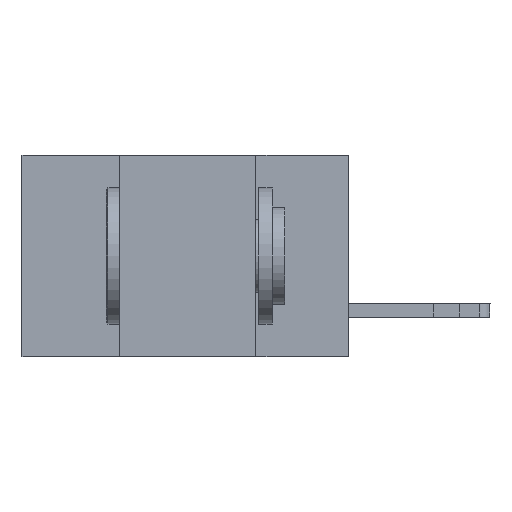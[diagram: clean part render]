
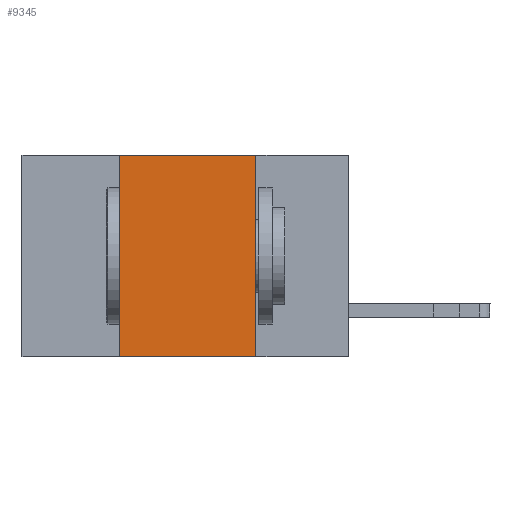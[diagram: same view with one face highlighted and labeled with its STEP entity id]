
A CAD part, left-side view. The second image highlights one B-rep face of the part: STEP entity #9345.
In plain terms, the highlighted planar face has unit normal (-1, 0, 0).
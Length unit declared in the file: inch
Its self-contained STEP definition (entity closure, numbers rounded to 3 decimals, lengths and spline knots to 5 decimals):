
#366 = AXIS2_PLACEMENT_3D ( 'NONE', #1109, #11660, #3903 ) ;
#400 = VECTOR ( 'NONE', #14167, 39.37008 ) ;
#1109 = CARTESIAN_POINT ( 'NONE',  ( 0., 0.6, 0. ) ) ;
#1203 = ORIENTED_EDGE ( 'NONE', *, *, #15492, .F. ) ;
#1875 = LINE ( 'NONE', #2284, #11899 ) ;
#2284 = CARTESIAN_POINT ( 'NONE',  ( 0., 0.6, -0.37 ) ) ;
#2560 = CARTESIAN_POINT ( 'NONE',  ( 0., 0.42, -0.37 ) ) ;
#3199 = DIRECTION ( 'NONE',  ( 0., 0., -1. ) ) ;
#3467 = CARTESIAN_POINT ( 'NONE',  ( 0., 0.17, -0.37 ) ) ;
#3658 = DIRECTION ( 'NONE',  ( 0., -1., 0. ) ) ;
#3903 = DIRECTION ( 'NONE',  ( 0., 0., -1. ) ) ;
#5061 = EDGE_CURVE ( 'NONE', #11461, #10512, #1875, .T. ) ;
#5116 = LINE ( 'NONE', #13193, #14806 ) ;
#6816 = EDGE_CURVE ( 'NONE', #8531, #10512, #14740, .T. ) ;
#8365 = ORIENTED_EDGE ( 'NONE', *, *, #14711, .F. ) ;
#8531 = VERTEX_POINT ( 'NONE', #12398 ) ;
#8611 = CARTESIAN_POINT ( 'NONE',  ( 0., 0.42, 0. ) ) ;
#9345 = ADVANCED_FACE ( 'NONE', ( #14860 ), #16462, .F. ) ;
#10512 = VERTEX_POINT ( 'NONE', #3467 ) ;
#10978 = CARTESIAN_POINT ( 'NONE',  ( 0., 0.17, -0.37 ) ) ;
#11001 = LINE ( 'NONE', #12928, #400 ) ;
#11461 = VERTEX_POINT ( 'NONE', #2560 ) ;
#11660 = DIRECTION ( 'NONE',  ( 1., 0., 0. ) ) ;
#11835 = VECTOR ( 'NONE', #3199, 39.37008 ) ;
#11899 = VECTOR ( 'NONE', #3658, 39.37008 ) ;
#12398 = CARTESIAN_POINT ( 'NONE',  ( 0., 0.17, 0. ) ) ;
#12705 = ORIENTED_EDGE ( 'NONE', *, *, #6816, .F. ) ;
#12928 = CARTESIAN_POINT ( 'NONE',  ( 0., 0.6, 0. ) ) ;
#12959 = ORIENTED_EDGE ( 'NONE', *, *, #5061, .T. ) ;
#13193 = CARTESIAN_POINT ( 'NONE',  ( 0., 0.42, -0.37 ) ) ;
#14167 = DIRECTION ( 'NONE',  ( 0., -1., 0. ) ) ;
#14418 = DIRECTION ( 'NONE',  ( 0., 0., 1. ) ) ;
#14518 = VERTEX_POINT ( 'NONE', #8611 ) ;
#14711 = EDGE_CURVE ( 'NONE', #14518, #8531, #11001, .T. ) ;
#14740 = LINE ( 'NONE', #10978, #11835 ) ;
#14806 = VECTOR ( 'NONE', #14418, 39.37008 ) ;
#14860 = FACE_OUTER_BOUND ( 'NONE', #15083, .T. ) ;
#15083 = EDGE_LOOP ( 'NONE', ( #12705, #8365, #1203, #12959 ) ) ;
#15492 = EDGE_CURVE ( 'NONE', #11461, #14518, #5116, .T. ) ;
#16462 = PLANE ( 'NONE',  #366 ) ;
